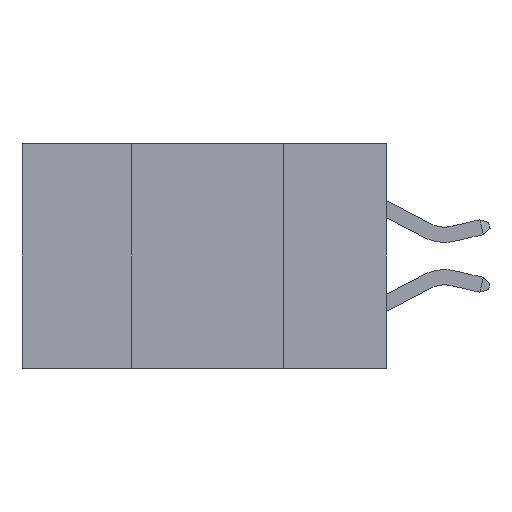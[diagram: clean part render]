
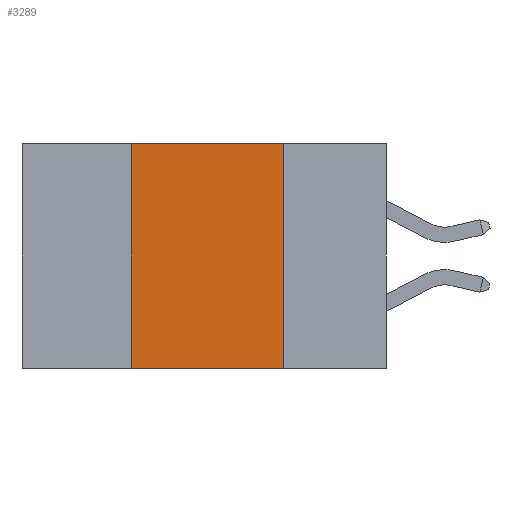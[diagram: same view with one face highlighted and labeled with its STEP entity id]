
A CAD part, left-side view. The second image highlights one B-rep face of the part: STEP entity #3289.
In plain terms, the highlighted planar face has unit normal (-1, 0, 0).
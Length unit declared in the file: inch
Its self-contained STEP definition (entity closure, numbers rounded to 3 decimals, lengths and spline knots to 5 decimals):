
#205 = VECTOR ( 'NONE', #8230, 39.37008 ) ;
#530 = EDGE_CURVE ( 'NONE', #21960, #25142, #7658, .T. ) ;
#1808 = ORIENTED_EDGE ( 'NONE', *, *, #9078, .F. ) ;
#2542 = ORIENTED_EDGE ( 'NONE', *, *, #14693, .F. ) ;
#3289 = ADVANCED_FACE ( 'NONE', ( #17526 ), #19875, .F. ) ;
#3589 = VECTOR ( 'NONE', #24691, 39.37008 ) ;
#3602 = DIRECTION ( 'NONE',  ( 0., -1., 0. ) ) ;
#6501 = CARTESIAN_POINT ( 'NONE',  ( 0., 0.17, 0. ) ) ;
#6630 = CARTESIAN_POINT ( 'NONE',  ( 0., 0.42, -0.37 ) ) ;
#6655 = VERTEX_POINT ( 'NONE', #6501 ) ;
#7658 = LINE ( 'NONE', #15645, #20502 ) ;
#7824 = DIRECTION ( 'NONE',  ( 1., 0., 0. ) ) ;
#8230 = DIRECTION ( 'NONE',  ( 0., -1., 0. ) ) ;
#8457 = DIRECTION ( 'NONE',  ( 0., 0., 1. ) ) ;
#9078 = EDGE_CURVE ( 'NONE', #16058, #6655, #16222, .T. ) ;
#11623 = DIRECTION ( 'NONE',  ( 0., 0., -1. ) ) ;
#12044 = EDGE_LOOP ( 'NONE', ( #2542, #1808, #24631, #24482 ) ) ;
#13708 = CARTESIAN_POINT ( 'NONE',  ( 0., 0.6, 0. ) ) ;
#13967 = CARTESIAN_POINT ( 'NONE',  ( 0., 0.6, 0. ) ) ;
#14194 = LINE ( 'NONE', #14585, #3589 ) ;
#14585 = CARTESIAN_POINT ( 'NONE',  ( 0., 0.17, -0.37 ) ) ;
#14693 = EDGE_CURVE ( 'NONE', #6655, #25142, #14194, .T. ) ;
#15602 = CARTESIAN_POINT ( 'NONE',  ( 0., 0.42, 0. ) ) ;
#15645 = CARTESIAN_POINT ( 'NONE',  ( 0., 0.6, -0.37 ) ) ;
#16058 = VERTEX_POINT ( 'NONE', #15602 ) ;
#16222 = LINE ( 'NONE', #13967, #205 ) ;
#17387 = EDGE_CURVE ( 'NONE', #21960, #16058, #24584, .T. ) ;
#17526 = FACE_OUTER_BOUND ( 'NONE', #12044, .T. ) ;
#19324 = CARTESIAN_POINT ( 'NONE',  ( 0., 0.17, -0.37 ) ) ;
#19875 = PLANE ( 'NONE',  #23324 ) ;
#19930 = VECTOR ( 'NONE', #8457, 39.37008 ) ;
#20502 = VECTOR ( 'NONE', #3602, 39.37008 ) ;
#21960 = VERTEX_POINT ( 'NONE', #25554 ) ;
#23324 = AXIS2_PLACEMENT_3D ( 'NONE', #13708, #7824, #11623 ) ;
#24482 = ORIENTED_EDGE ( 'NONE', *, *, #530, .T. ) ;
#24584 = LINE ( 'NONE', #6630, #19930 ) ;
#24631 = ORIENTED_EDGE ( 'NONE', *, *, #17387, .F. ) ;
#24691 = DIRECTION ( 'NONE',  ( 0., 0., -1. ) ) ;
#25142 = VERTEX_POINT ( 'NONE', #19324 ) ;
#25554 = CARTESIAN_POINT ( 'NONE',  ( 0., 0.42, -0.37 ) ) ;
